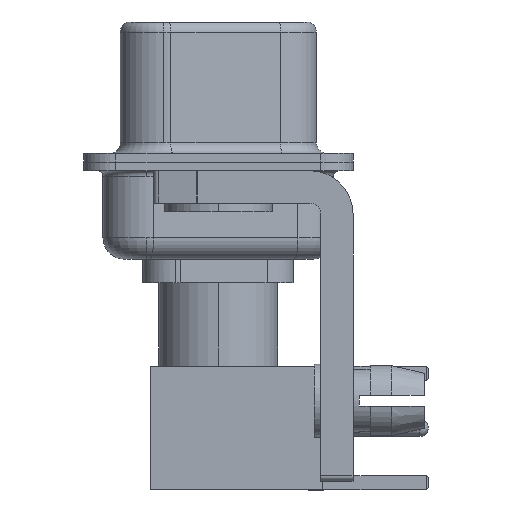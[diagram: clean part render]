
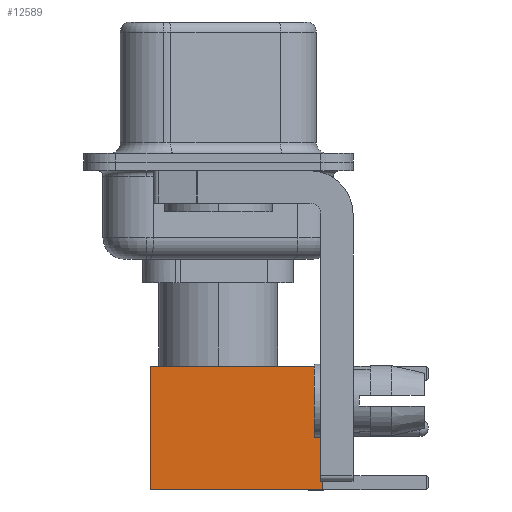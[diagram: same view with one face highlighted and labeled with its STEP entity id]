
A CAD part, left-side view. The second image highlights one B-rep face of the part: STEP entity #12589.
In plain terms, the highlighted face is planar.
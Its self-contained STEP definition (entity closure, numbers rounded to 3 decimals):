
#354 = EDGE_CURVE ( 'NONE', #4309, #7076, #11314, .T. ) ;
#2472 = ORIENTED_EDGE ( 'NONE', *, *, #10188, .T. ) ;
#3170 = ORIENTED_EDGE ( 'NONE', *, *, #354, .F. ) ;
#3362 = VERTEX_POINT ( 'NONE', #18327 ) ;
#3533 = LINE ( 'NONE', #13920, #17923 ) ;
#4271 = FACE_OUTER_BOUND ( 'NONE', #5042, .T. ) ;
#4309 = VERTEX_POINT ( 'NONE', #5999 ) ;
#5042 = EDGE_LOOP ( 'NONE', ( #13008, #2472, #5312, #3170 ) ) ;
#5312 = ORIENTED_EDGE ( 'NONE', *, *, #13295, .F. ) ;
#5899 = DIRECTION ( 'NONE',  ( -1., 0., 0. ) ) ;
#5999 = CARTESIAN_POINT ( 'NONE',  ( 2.875, 2.875, 8. ) ) ;
#6898 = CARTESIAN_POINT ( 'NONE',  ( -2.875, 2.875, 8. ) ) ;
#7076 = VERTEX_POINT ( 'NONE', #6898 ) ;
#7394 = DIRECTION ( 'NONE',  ( 0., 0., 1. ) ) ;
#7588 = DIRECTION ( 'NONE',  ( 0., 1., 0. ) ) ;
#8149 = DIRECTION ( 'NONE',  ( 0., 0., -1. ) ) ;
#8630 = LINE ( 'NONE', #11967, #18764 ) ;
#8810 = CARTESIAN_POINT ( 'NONE',  ( -2.875, 2.875, 0. ) ) ;
#10188 = EDGE_CURVE ( 'NONE', #3362, #10523, #8630, .T. ) ;
#10420 = CARTESIAN_POINT ( 'NONE',  ( 2.875, 2.875, 0. ) ) ;
#10523 = VERTEX_POINT ( 'NONE', #8810 ) ;
#11314 = LINE ( 'NONE', #14330, #14422 ) ;
#11516 = DIRECTION ( 'NONE',  ( -1., 0., 0. ) ) ;
#11967 = CARTESIAN_POINT ( 'NONE',  ( 0., 2.875, 0. ) ) ;
#12589 = ADVANCED_FACE ( 'NONE', ( #4271 ), #19559, .T. ) ;
#13008 = ORIENTED_EDGE ( 'NONE', *, *, #16246, .T. ) ;
#13295 = EDGE_CURVE ( 'NONE', #7076, #10523, #3533, .T. ) ;
#13920 = CARTESIAN_POINT ( 'NONE',  ( -2.875, 2.875, 0. ) ) ;
#14330 = CARTESIAN_POINT ( 'NONE',  ( 0., 2.875, 8. ) ) ;
#14422 = VECTOR ( 'NONE', #11516, 1000. ) ;
#15590 = LINE ( 'NONE', #15791, #18219 ) ;
#15791 = CARTESIAN_POINT ( 'NONE',  ( 2.875, 2.875, 0. ) ) ;
#16246 = EDGE_CURVE ( 'NONE', #4309, #3362, #15590, .T. ) ;
#17923 = VECTOR ( 'NONE', #8149, 1000. ) ;
#18212 = AXIS2_PLACEMENT_3D ( 'NONE', #10420, #7588, #7394 ) ;
#18219 = VECTOR ( 'NONE', #18993, 1000. ) ;
#18327 = CARTESIAN_POINT ( 'NONE',  ( 2.875, 2.875, 0. ) ) ;
#18764 = VECTOR ( 'NONE', #5899, 1000. ) ;
#18993 = DIRECTION ( 'NONE',  ( 0., 0., -1. ) ) ;
#19559 = PLANE ( 'NONE',  #18212 ) ;
